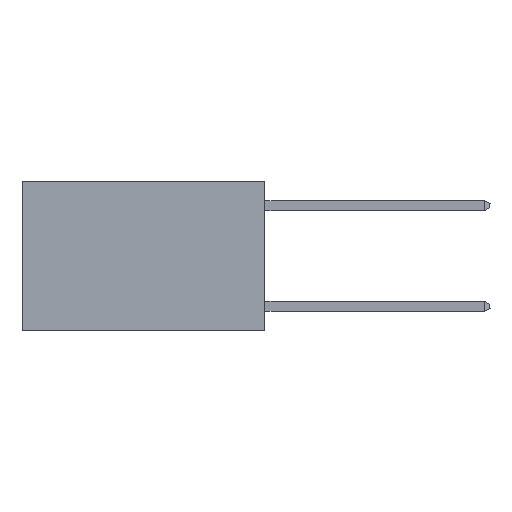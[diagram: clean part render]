
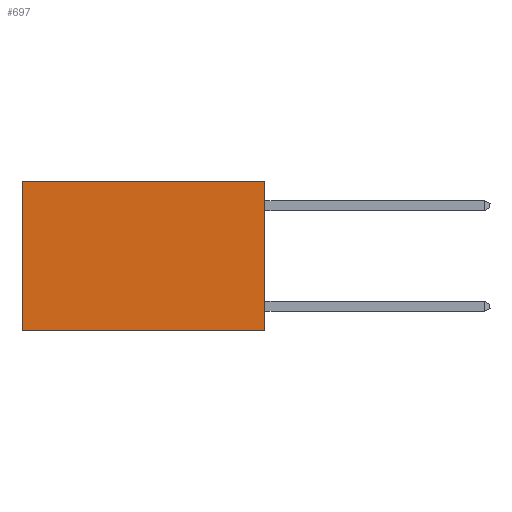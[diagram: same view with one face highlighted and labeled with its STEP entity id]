
A CAD part, left-side view. The second image highlights one B-rep face of the part: STEP entity #697.
In plain terms, the highlighted planar face has unit normal (-1, 0, 0).
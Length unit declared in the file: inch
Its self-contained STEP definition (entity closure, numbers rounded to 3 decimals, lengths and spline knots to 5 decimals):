
#420 = CARTESIAN_POINT ( 'NONE',  ( 0.2625, 0., -0.37 ) ) ;
#697 = ADVANCED_FACE ( 'NONE', ( #1003 ), #18539, .F. ) ;
#1003 = FACE_OUTER_BOUND ( 'NONE', #3192, .T. ) ;
#2103 = DIRECTION ( 'NONE',  ( 0., 0., -1. ) ) ;
#2220 = LINE ( 'NONE', #6640, #11650 ) ;
#2302 = ORIENTED_EDGE ( 'NONE', *, *, #15139, .T. ) ;
#2390 = VERTEX_POINT ( 'NONE', #13340 ) ;
#3192 = EDGE_LOOP ( 'NONE', ( #2302, #11465, #17405, #3424 ) ) ;
#3424 = ORIENTED_EDGE ( 'NONE', *, *, #17255, .T. ) ;
#4188 = LINE ( 'NONE', #8504, #6885 ) ;
#5036 = DIRECTION ( 'NONE',  ( 0., 0., -1. ) ) ;
#6640 = CARTESIAN_POINT ( 'NONE',  ( 0.2625, 0., 0. ) ) ;
#6885 = VECTOR ( 'NONE', #15982, 39.37008 ) ;
#8172 = LINE ( 'NONE', #18512, #12862 ) ;
#8504 = CARTESIAN_POINT ( 'NONE',  ( 0.2625, 0., 0. ) ) ;
#10351 = VERTEX_POINT ( 'NONE', #420 ) ;
#10389 = VERTEX_POINT ( 'NONE', #17022 ) ;
#11433 = DIRECTION ( 'NONE',  ( 1., 0., 0. ) ) ;
#11465 = ORIENTED_EDGE ( 'NONE', *, *, #14626, .F. ) ;
#11650 = VECTOR ( 'NONE', #18967, 39.37008 ) ;
#12862 = VECTOR ( 'NONE', #5036, 39.37008 ) ;
#13042 = CARTESIAN_POINT ( 'NONE',  ( 0.2625, 0., -0.37 ) ) ;
#13340 = CARTESIAN_POINT ( 'NONE',  ( 0.2625, 0.6, 0. ) ) ;
#14477 = CARTESIAN_POINT ( 'NONE',  ( 0.2625, 0., 0. ) ) ;
#14626 = EDGE_CURVE ( 'NONE', #10351, #10389, #15760, .T. ) ;
#15139 = EDGE_CURVE ( 'NONE', #2390, #10389, #8172, .T. ) ;
#15460 = AXIS2_PLACEMENT_3D ( 'NONE', #14477, #11433, #2103 ) ;
#15760 = LINE ( 'NONE', #13042, #16910 ) ;
#15939 = EDGE_CURVE ( 'NONE', #19336, #10351, #4188, .T. ) ;
#15982 = DIRECTION ( 'NONE',  ( 0., 0., -1. ) ) ;
#16652 = CARTESIAN_POINT ( 'NONE',  ( 0.2625, 0., 0. ) ) ;
#16910 = VECTOR ( 'NONE', #18636, 39.37008 ) ;
#17022 = CARTESIAN_POINT ( 'NONE',  ( 0.2625, 0.6, -0.37 ) ) ;
#17255 = EDGE_CURVE ( 'NONE', #19336, #2390, #2220, .T. ) ;
#17405 = ORIENTED_EDGE ( 'NONE', *, *, #15939, .F. ) ;
#18512 = CARTESIAN_POINT ( 'NONE',  ( 0.2625, 0.6, 0. ) ) ;
#18539 = PLANE ( 'NONE',  #15460 ) ;
#18636 = DIRECTION ( 'NONE',  ( 0., 1., 0. ) ) ;
#18967 = DIRECTION ( 'NONE',  ( 0., 1., 0. ) ) ;
#19336 = VERTEX_POINT ( 'NONE', #16652 ) ;
